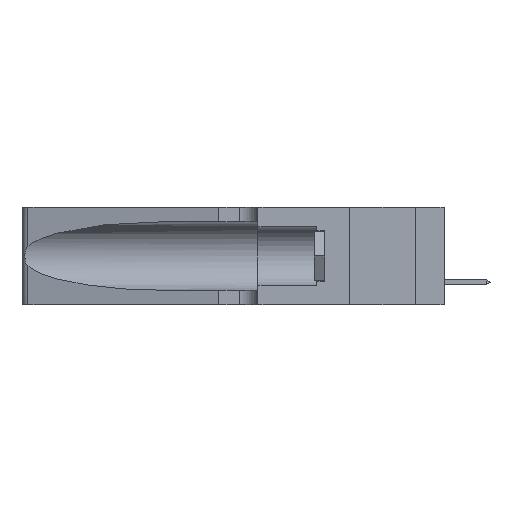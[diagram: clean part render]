
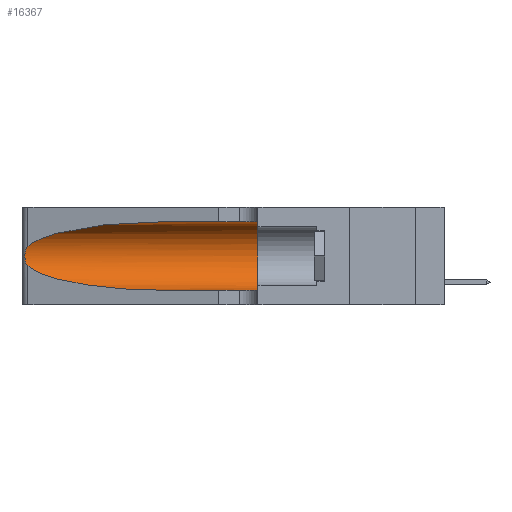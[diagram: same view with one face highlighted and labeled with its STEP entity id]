
A CAD part, left-side view. The second image highlights one B-rep face of the part: STEP entity #16367.
In plain terms, the highlighted cylindrical face has radius 3.308 mm (diameter 6.617 mm), a partial arc.
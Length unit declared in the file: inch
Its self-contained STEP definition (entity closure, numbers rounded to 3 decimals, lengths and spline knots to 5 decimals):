
#140 = CARTESIAN_POINT ( 'NONE',  ( 0.25639, 1.23184, 0.21858 ) ) ;
#231 = CARTESIAN_POINT ( 'NONE',  ( 0.1305, 1.61858, 0.05475 ) ) ;
#326 = CARTESIAN_POINT ( 'NONE',  ( 0.26018, 1.23835, 0.19895 ) ) ;
#626 = EDGE_LOOP ( 'NONE', ( #5981, #684, #12188, #13844, #1794, #11720 ) ) ;
#684 = ORIENTED_EDGE ( 'NONE', *, *, #12809, .T. ) ;
#747 = FACE_OUTER_BOUND ( 'NONE', #626, .T. ) ;
#1292 = CARTESIAN_POINT ( 'NONE',  ( 0.25487, 1.22718, 0.14631 ) ) ;
#1395 = AXIS2_PLACEMENT_3D ( 'NONE', #7953, #15188, #3871 ) ;
#1574 = CARTESIAN_POINT ( 'NONE',  ( 0.25854, 1.2359, 0.20912 ) ) ;
#1794 = ORIENTED_EDGE ( 'NONE', *, *, #10345, .F. ) ;
#1997 =( BOUNDED_CURVE ( )  B_SPLINE_CURVE ( 3, ( #1292, #15779, #2931, #11350 ),
 .UNSPECIFIED., .F., .T. ) 
 B_SPLINE_CURVE_WITH_KNOTS ( ( 4, 4 ),
 ( 3.44316, 4.71239 ),
 .UNSPECIFIED. ) 
 CURVE ( )  GEOMETRIC_REPRESENTATION_ITEM ( )  RATIONAL_B_SPLINE_CURVE ( ( 1., 0.87, 0.87, 1. ) ) 
 REPRESENTATION_ITEM ( '' )  );
#2896 = DIRECTION ( 'NONE',  ( 0., -1., 0. ) ) ;
#2931 = CARTESIAN_POINT ( 'NONE',  ( 0.18966, 0.96281, 0.05475 ) ) ;
#2975 = CARTESIAN_POINT ( 'NONE',  ( 0.25487, 1.22718, 0.22369 ) ) ;
#3783 = EDGE_CURVE ( 'NONE', #18072, #7547, #1997, .T. ) ;
#3871 = DIRECTION ( 'NONE',  ( 0., 0., 1. ) ) ;
#4239 = LINE ( 'NONE', #231, #8032 ) ;
#5244 = CARTESIAN_POINT ( 'NONE',  ( 0.2373, 1.15595, 0.28018 ) ) ;
#5290 = DIRECTION ( 'NONE',  ( 0., -1., 0. ) ) ;
#5482 = EDGE_CURVE ( 'NONE', #7547, #11952, #4239, .T. ) ;
#5535 = CARTESIAN_POINT ( 'NONE',  ( 0.25487, 1.22718, 0.22369 ) ) ;
#5664 = CARTESIAN_POINT ( 'NONE',  ( 0.1305, 0.35, 0.31525 ) ) ;
#5741 = VERTEX_POINT ( 'NONE', #5664 ) ;
#5868 = CARTESIAN_POINT ( 'NONE',  ( 0.25856, 1.23593, 0.16098 ) ) ;
#5928 = CARTESIAN_POINT ( 'NONE',  ( 0.1305, 1.61858, 0.185 ) ) ;
#5936 = CARTESIAN_POINT ( 'NONE',  ( 0.25487, 1.22718, 0.14631 ) ) ;
#5981 = ORIENTED_EDGE ( 'NONE', *, *, #10058, .T. ) ;
#5990 = DIRECTION ( 'NONE',  ( 0., 0., -1. ) ) ;
#7501 = CARTESIAN_POINT ( 'NONE',  ( 0.25787, 1.23484, 0.2124 ) ) ;
#7547 = VERTEX_POINT ( 'NONE', #10069 ) ;
#7559 = CARTESIAN_POINT ( 'NONE',  ( 0.25639, 1.23186, 0.15144 ) ) ;
#7663 =( BOUNDED_CURVE ( )  B_SPLINE_CURVE ( 3, ( #15415, #18178, #5244, #12416 ),
 .UNSPECIFIED., .F., .T. ) 
 B_SPLINE_CURVE_WITH_KNOTS ( ( 4, 4 ),
 ( 1.5708, 2.84003 ),
 .UNSPECIFIED. ) 
 CURVE ( )  GEOMETRIC_REPRESENTATION_ITEM ( )  RATIONAL_B_SPLINE_CURVE ( ( 1., 0.87, 0.87, 1. ) ) 
 REPRESENTATION_ITEM ( '' )  );
#7953 = CARTESIAN_POINT ( 'NONE',  ( 0.1305, 0.35, 0.185 ) ) ;
#8032 = VECTOR ( 'NONE', #14773, 39.37008 ) ;
#8381 = VERTEX_POINT ( 'NONE', #17621 ) ;
#8409 = CYLINDRICAL_SURFACE ( 'NONE', #16971, 0.13025 ) ;
#8742 = LINE ( 'NONE', #11000, #10281 ) ;
#8920 = CARTESIAN_POINT ( 'NONE',  ( 0.26075, 1.23896, 0.178 ) ) ;
#10058 = EDGE_CURVE ( 'NONE', #8381, #16951, #7663, .T. ) ;
#10069 = CARTESIAN_POINT ( 'NONE',  ( 0.1305, 0.72297, 0.05475 ) ) ;
#10167 = CARTESIAN_POINT ( 'NONE',  ( 0.25555, 1.22993, 0.14849 ) ) ;
#10281 = VECTOR ( 'NONE', #5290, 39.37008 ) ;
#10290 = CARTESIAN_POINT ( 'NONE',  ( 0.26017, 1.23833, 0.17102 ) ) ;
#10345 = EDGE_CURVE ( 'NONE', #5741, #11952, #12620, .T. ) ;
#11000 = CARTESIAN_POINT ( 'NONE',  ( 0.1305, 1.61858, 0.31525 ) ) ;
#11350 = CARTESIAN_POINT ( 'NONE',  ( 0.1305, 0.72297, 0.05475 ) ) ;
#11720 = ORIENTED_EDGE ( 'NONE', *, *, #13130, .F. ) ;
#11767 = CARTESIAN_POINT ( 'NONE',  ( 0.26075, 1.23896, 0.19203 ) ) ;
#11952 = VERTEX_POINT ( 'NONE', #16715 ) ;
#12188 = ORIENTED_EDGE ( 'NONE', *, *, #3783, .T. ) ;
#12416 = CARTESIAN_POINT ( 'NONE',  ( 0.25487, 1.22718, 0.22369 ) ) ;
#12564 = B_SPLINE_CURVE_WITH_KNOTS ( 'NONE', 3,
 ( #2975, #18432, #140, #7501, #1574, #326, #11767, #8920, #10290, #5868, #15890, #7559, #10167, #5936 ),
 .UNSPECIFIED., .F., .F.,
 ( 4, 2, 2, 2, 2, 2, 4 ),
 ( 0., 0.00027, 0.00053, 0.00107, 0.0016, 0.00187, 0.00214 ),
 .UNSPECIFIED. ) ;
#12620 = CIRCLE ( 'NONE', #1395, 0.13025 ) ;
#12809 = EDGE_CURVE ( 'NONE', #16951, #18072, #12564, .T. ) ;
#13130 = EDGE_CURVE ( 'NONE', #8381, #5741, #8742, .T. ) ;
#13844 = ORIENTED_EDGE ( 'NONE', *, *, #5482, .T. ) ;
#14773 = DIRECTION ( 'NONE',  ( 0., -1., 0. ) ) ;
#15188 = DIRECTION ( 'NONE',  ( 0., 1., 0. ) ) ;
#15415 = CARTESIAN_POINT ( 'NONE',  ( 0.1305, 0.72297, 0.31525 ) ) ;
#15779 = CARTESIAN_POINT ( 'NONE',  ( 0.2373, 1.15595, 0.08982 ) ) ;
#15890 = CARTESIAN_POINT ( 'NONE',  ( 0.25789, 1.23486, 0.15765 ) ) ;
#16367 = ADVANCED_FACE ( 'NONE', ( #747 ), #8409, .F. ) ;
#16561 = CARTESIAN_POINT ( 'NONE',  ( 0.25487, 1.22718, 0.14631 ) ) ;
#16715 = CARTESIAN_POINT ( 'NONE',  ( 0.1305, 0.35, 0.05475 ) ) ;
#16951 = VERTEX_POINT ( 'NONE', #5535 ) ;
#16971 = AXIS2_PLACEMENT_3D ( 'NONE', #5928, #2896, #5990 ) ;
#17621 = CARTESIAN_POINT ( 'NONE',  ( 0.1305, 0.72297, 0.31525 ) ) ;
#18072 = VERTEX_POINT ( 'NONE', #16561 ) ;
#18178 = CARTESIAN_POINT ( 'NONE',  ( 0.18966, 0.96281, 0.31525 ) ) ;
#18432 = CARTESIAN_POINT ( 'NONE',  ( 0.25555, 1.22994, 0.2215 ) ) ;
